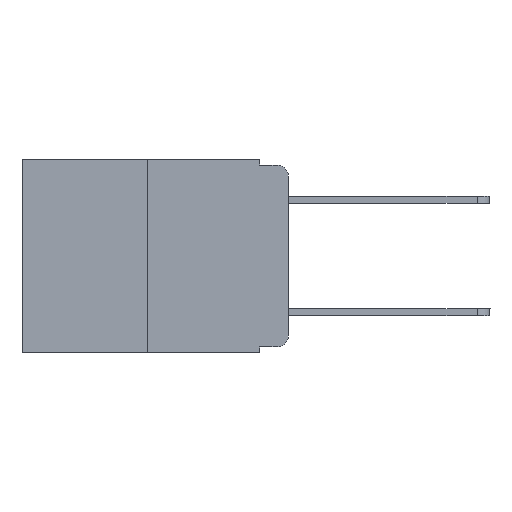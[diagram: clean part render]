
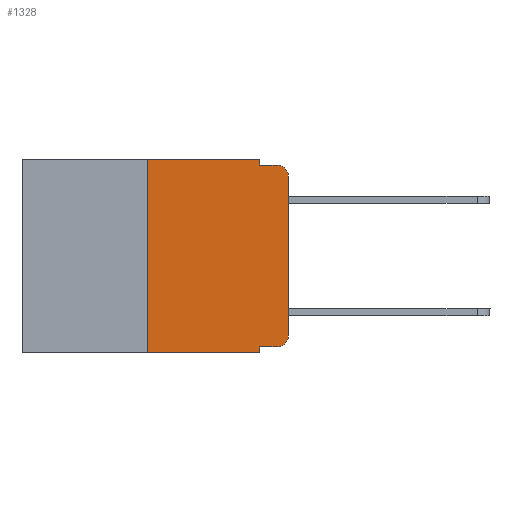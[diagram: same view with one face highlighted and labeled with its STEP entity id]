
A CAD part, left-side view. The second image highlights one B-rep face of the part: STEP entity #1328.
In plain terms, the highlighted planar face has unit normal (-1, 0, 0).
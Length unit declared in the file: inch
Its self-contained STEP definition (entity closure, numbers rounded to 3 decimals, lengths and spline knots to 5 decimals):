
#354 = CARTESIAN_POINT ( 'NONE',  ( 0., 0.051, -0.01 ) ) ;
#365 = VERTEX_POINT ( 'NONE', #12700 ) ;
#710 = LINE ( 'NONE', #10578, #3232 ) ;
#1102 = ORIENTED_EDGE ( 'NONE', *, *, #4635, .F. ) ;
#1133 = DIRECTION ( 'NONE',  ( 0., 0., -1. ) ) ;
#1258 = ORIENTED_EDGE ( 'NONE', *, *, #8779, .F. ) ;
#1328 = ADVANCED_FACE ( 'NONE', ( #6578 ), #12268, .F. ) ;
#1719 = VECTOR ( 'NONE', #4855, 39.37008 ) ;
#1879 = EDGE_CURVE ( 'NONE', #5812, #10864, #8582, .T. ) ;
#1945 = EDGE_CURVE ( 'NONE', #10938, #12668, #10269, .T. ) ;
#2122 = ORIENTED_EDGE ( 'NONE', *, *, #7114, .T. ) ;
#2338 = DIRECTION ( 'NONE',  ( 0., 0., 1. ) ) ;
#2549 = CARTESIAN_POINT ( 'NONE',  ( 0., 0.051, -0.333 ) ) ;
#2638 = DIRECTION ( 'NONE',  ( 0., -1., 0. ) ) ;
#3232 = VECTOR ( 'NONE', #12495, 39.37008 ) ;
#3265 = ORIENTED_EDGE ( 'NONE', *, *, #8569, .T. ) ;
#3289 = ORIENTED_EDGE ( 'NONE', *, *, #13717, .T. ) ;
#3485 = VECTOR ( 'NONE', #2338, 39.37008 ) ;
#3587 = VERTEX_POINT ( 'NONE', #8603 ) ;
#3695 = ORIENTED_EDGE ( 'NONE', *, *, #1879, .F. ) ;
#3776 = CARTESIAN_POINT ( 'NONE',  ( 0., 0.02, -0.01 ) ) ;
#3865 = CARTESIAN_POINT ( 'NONE',  ( 0., 0.051, 0. ) ) ;
#4171 = VECTOR ( 'NONE', #13593, 39.37008 ) ;
#4635 = EDGE_CURVE ( 'NONE', #10492, #7249, #7683, .T. ) ;
#4855 = DIRECTION ( 'NONE',  ( 0., -1., 0. ) ) ;
#5084 = DIRECTION ( 'NONE',  ( -1., 0., 0. ) ) ;
#5366 = VECTOR ( 'NONE', #13543, 39.37008 ) ;
#5408 = CIRCLE ( 'NONE', #10170, 0.02 ) ;
#5676 = AXIS2_PLACEMENT_3D ( 'NONE', #12166, #11067, #5728 ) ;
#5728 = DIRECTION ( 'NONE',  ( 0., 0., -1. ) ) ;
#5800 = LINE ( 'NONE', #2549, #1719 ) ;
#5812 = VERTEX_POINT ( 'NONE', #7076 ) ;
#6106 = CARTESIAN_POINT ( 'NONE',  ( 0., 0., 0. ) ) ;
#6133 = CARTESIAN_POINT ( 'NONE',  ( 0., 0.473, 0. ) ) ;
#6560 = CARTESIAN_POINT ( 'NONE',  ( 0., 0.02, -0.03 ) ) ;
#6578 = FACE_OUTER_BOUND ( 'NONE', #13212, .T. ) ;
#6783 = CIRCLE ( 'NONE', #12498, 0.02 ) ;
#7076 = CARTESIAN_POINT ( 'NONE',  ( 0., 0.25, -0.343 ) ) ;
#7114 = EDGE_CURVE ( 'NONE', #13754, #12924, #11065, .T. ) ;
#7249 = VERTEX_POINT ( 'NONE', #3776 ) ;
#7488 = LINE ( 'NONE', #6133, #11877 ) ;
#7642 = DIRECTION ( 'NONE',  ( -1., 0., 0. ) ) ;
#7683 = LINE ( 'NONE', #8124, #9538 ) ;
#7685 = CARTESIAN_POINT ( 'NONE',  ( 0., 0.25, 0. ) ) ;
#7814 = ORIENTED_EDGE ( 'NONE', *, *, #10422, .T. ) ;
#7985 = ORIENTED_EDGE ( 'NONE', *, *, #1945, .F. ) ;
#8124 = CARTESIAN_POINT ( 'NONE',  ( 0., 0.051, -0.01 ) ) ;
#8349 = EDGE_CURVE ( 'NONE', #5812, #12668, #710, .T. ) ;
#8380 = DIRECTION ( 'NONE',  ( 0., 0., -1. ) ) ;
#8569 = EDGE_CURVE ( 'NONE', #10938, #365, #5800, .T. ) ;
#8582 = LINE ( 'NONE', #7685, #3485 ) ;
#8603 = CARTESIAN_POINT ( 'NONE',  ( 0., 0.051, 0. ) ) ;
#8779 = EDGE_CURVE ( 'NONE', #10864, #3587, #7488, .T. ) ;
#8867 = VECTOR ( 'NONE', #13668, 39.37008 ) ;
#9417 = CARTESIAN_POINT ( 'NONE',  ( 0., 0.02, -0.313 ) ) ;
#9538 = VECTOR ( 'NONE', #10284, 39.37008 ) ;
#10018 = CARTESIAN_POINT ( 'NONE',  ( 0., 0.051, 0. ) ) ;
#10170 = AXIS2_PLACEMENT_3D ( 'NONE', #6560, #7642, #1133 ) ;
#10269 = LINE ( 'NONE', #10018, #5366 ) ;
#10284 = DIRECTION ( 'NONE',  ( 0., -1., 0. ) ) ;
#10422 = EDGE_CURVE ( 'NONE', #12924, #7249, #5408, .T. ) ;
#10492 = VERTEX_POINT ( 'NONE', #354 ) ;
#10578 = CARTESIAN_POINT ( 'NONE',  ( 0., 0.473, -0.343 ) ) ;
#10599 = CARTESIAN_POINT ( 'NONE',  ( 0., 0., -0.313 ) ) ;
#10810 = CARTESIAN_POINT ( 'NONE',  ( 0., 0.051, -0.343 ) ) ;
#10864 = VERTEX_POINT ( 'NONE', #13740 ) ;
#10938 = VERTEX_POINT ( 'NONE', #12784 ) ;
#10944 = LINE ( 'NONE', #3865, #4171 ) ;
#11065 = LINE ( 'NONE', #6106, #8867 ) ;
#11067 = DIRECTION ( 'NONE',  ( 1., 0., 0. ) ) ;
#11143 = ORIENTED_EDGE ( 'NONE', *, *, #8349, .T. ) ;
#11287 = CARTESIAN_POINT ( 'NONE',  ( 0., 0., -0.03 ) ) ;
#11853 = EDGE_CURVE ( 'NONE', #3587, #10492, #10944, .T. ) ;
#11877 = VECTOR ( 'NONE', #2638, 39.37008 ) ;
#12166 = CARTESIAN_POINT ( 'NONE',  ( 0., 0.473, 0. ) ) ;
#12268 = PLANE ( 'NONE',  #5676 ) ;
#12495 = DIRECTION ( 'NONE',  ( 0., -1., 0. ) ) ;
#12498 = AXIS2_PLACEMENT_3D ( 'NONE', #9417, #5084, #8380 ) ;
#12668 = VERTEX_POINT ( 'NONE', #10810 ) ;
#12700 = CARTESIAN_POINT ( 'NONE',  ( 0., 0.02, -0.333 ) ) ;
#12784 = CARTESIAN_POINT ( 'NONE',  ( 0., 0.051, -0.333 ) ) ;
#12924 = VERTEX_POINT ( 'NONE', #11287 ) ;
#13212 = EDGE_LOOP ( 'NONE', ( #2122, #7814, #1102, #13846, #1258, #3695, #11143, #7985, #3265, #3289 ) ) ;
#13543 = DIRECTION ( 'NONE',  ( 0., 0., -1. ) ) ;
#13593 = DIRECTION ( 'NONE',  ( 0., 0., -1. ) ) ;
#13668 = DIRECTION ( 'NONE',  ( 0., 0., 1. ) ) ;
#13717 = EDGE_CURVE ( 'NONE', #365, #13754, #6783, .T. ) ;
#13740 = CARTESIAN_POINT ( 'NONE',  ( 0., 0.25, 0. ) ) ;
#13754 = VERTEX_POINT ( 'NONE', #10599 ) ;
#13846 = ORIENTED_EDGE ( 'NONE', *, *, #11853, .F. ) ;
